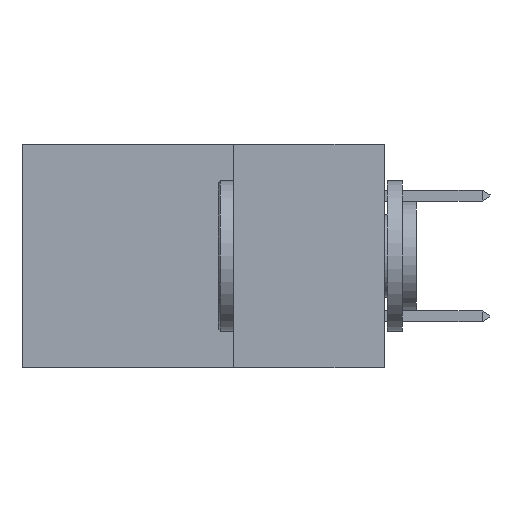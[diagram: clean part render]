
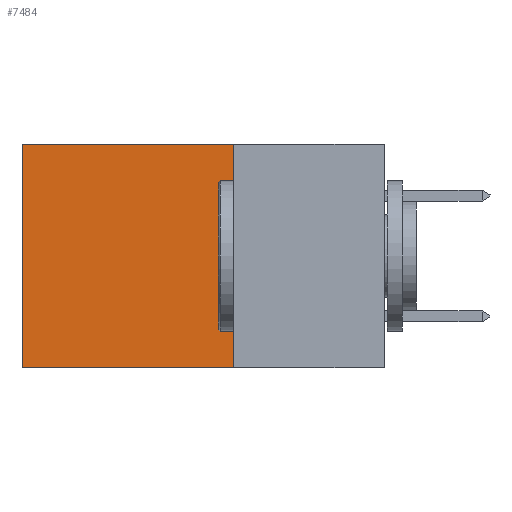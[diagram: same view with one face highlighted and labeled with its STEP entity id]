
A CAD part, left-side view. The second image highlights one B-rep face of the part: STEP entity #7484.
In plain terms, the highlighted planar face has unit normal (-1, 0, 0).
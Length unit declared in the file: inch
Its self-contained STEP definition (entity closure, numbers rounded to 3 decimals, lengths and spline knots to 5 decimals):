
#61 = LINE ( 'NONE', #13976, #11857 ) ;
#1975 = ORIENTED_EDGE ( 'NONE', *, *, #13480, .T. ) ;
#2584 = FACE_OUTER_BOUND ( 'NONE', #31475, .T. ) ;
#3290 = AXIS2_PLACEMENT_3D ( 'NONE', #27411, #29914, #14927 ) ;
#4221 = CARTESIAN_POINT ( 'NONE',  ( 0.2875, 0.25, -0.37 ) ) ;
#4743 = VERTEX_POINT ( 'NONE', #15582 ) ;
#5972 = VERTEX_POINT ( 'NONE', #8736 ) ;
#6822 = ORIENTED_EDGE ( 'NONE', *, *, #20522, .F. ) ;
#7484 = ADVANCED_FACE ( 'NONE', ( #2584 ), #9843, .F. ) ;
#8736 = CARTESIAN_POINT ( 'NONE',  ( 0.2875, 0.6, 0. ) ) ;
#9843 = PLANE ( 'NONE',  #3290 ) ;
#11046 = EDGE_CURVE ( 'NONE', #24980, #5972, #61, .T. ) ;
#11857 = VECTOR ( 'NONE', #26445, 39.37008 ) ;
#12081 = LINE ( 'NONE', #28292, #24644 ) ;
#13480 = EDGE_CURVE ( 'NONE', #5972, #4743, #12081, .T. ) ;
#13517 = CARTESIAN_POINT ( 'NONE',  ( 0.2875, 0.25, 0. ) ) ;
#13976 = CARTESIAN_POINT ( 'NONE',  ( 0.2875, 0.25, 0. ) ) ;
#14927 = DIRECTION ( 'NONE',  ( 0., 0., -1. ) ) ;
#15269 = CARTESIAN_POINT ( 'NONE',  ( 0.2875, 0.25, 0. ) ) ;
#15582 = CARTESIAN_POINT ( 'NONE',  ( 0.2875, 0.6, -0.37 ) ) ;
#15714 = DIRECTION ( 'NONE',  ( 0., 0., -1. ) ) ;
#15719 = VECTOR ( 'NONE', #25195, 39.37008 ) ;
#16802 = VECTOR ( 'NONE', #28510, 39.37008 ) ;
#18547 = ORIENTED_EDGE ( 'NONE', *, *, #11046, .T. ) ;
#19497 = ORIENTED_EDGE ( 'NONE', *, *, #25677, .F. ) ;
#20522 = EDGE_CURVE ( 'NONE', #24980, #29928, #29325, .T. ) ;
#24644 = VECTOR ( 'NONE', #15714, 39.37008 ) ;
#24980 = VERTEX_POINT ( 'NONE', #15269 ) ;
#25195 = DIRECTION ( 'NONE',  ( 0., 1., 0. ) ) ;
#25677 = EDGE_CURVE ( 'NONE', #29928, #4743, #29796, .T. ) ;
#26445 = DIRECTION ( 'NONE',  ( 0., 1., 0. ) ) ;
#27411 = CARTESIAN_POINT ( 'NONE',  ( 0.2875, 0.25, 0. ) ) ;
#27720 = CARTESIAN_POINT ( 'NONE',  ( 0.2875, 0.25, -0.37 ) ) ;
#28292 = CARTESIAN_POINT ( 'NONE',  ( 0.2875, 0.6, 0. ) ) ;
#28510 = DIRECTION ( 'NONE',  ( 0., 0., -1. ) ) ;
#29325 = LINE ( 'NONE', #13517, #16802 ) ;
#29796 = LINE ( 'NONE', #27720, #15719 ) ;
#29914 = DIRECTION ( 'NONE',  ( 1., 0., 0. ) ) ;
#29928 = VERTEX_POINT ( 'NONE', #4221 ) ;
#31475 = EDGE_LOOP ( 'NONE', ( #1975, #19497, #6822, #18547 ) ) ;
